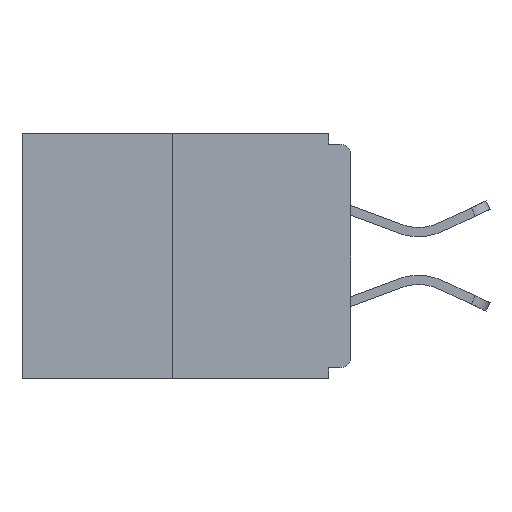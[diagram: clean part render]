
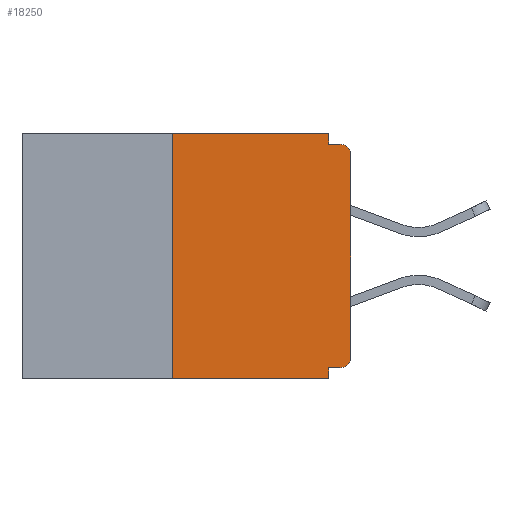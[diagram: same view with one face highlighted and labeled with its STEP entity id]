
A CAD part, left-side view. The second image highlights one B-rep face of the part: STEP entity #18250.
In plain terms, the highlighted planar face has unit normal (-1, 0, 0).
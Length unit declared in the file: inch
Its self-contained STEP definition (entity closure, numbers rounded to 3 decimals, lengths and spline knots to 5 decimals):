
#470 = CARTESIAN_POINT ( 'NONE',  ( 0., 0.46, 0. ) ) ;
#754 = AXIS2_PLACEMENT_3D ( 'NONE', #14094, #1315, #24975 ) ;
#1192 = VECTOR ( 'NONE', #9846, 39.37008 ) ;
#1315 = DIRECTION ( 'NONE',  ( -1., 0., 0. ) ) ;
#2148 = ORIENTED_EDGE ( 'NONE', *, *, #24529, .T. ) ;
#2165 = ORIENTED_EDGE ( 'NONE', *, *, #6232, .F. ) ;
#2909 = DIRECTION ( 'NONE',  ( 1., 0., 0. ) ) ;
#2956 = DIRECTION ( 'NONE',  ( 0., 1., 0. ) ) ;
#3475 = VERTEX_POINT ( 'NONE', #12424 ) ;
#3499 = CARTESIAN_POINT ( 'NONE',  ( 0., 0., 0. ) ) ;
#3639 = ORIENTED_EDGE ( 'NONE', *, *, #13414, .F. ) ;
#4383 = VERTEX_POINT ( 'NONE', #13412 ) ;
#4869 = ORIENTED_EDGE ( 'NONE', *, *, #10185, .T. ) ;
#4940 = CARTESIAN_POINT ( 'NONE',  ( 0., 0., -0.328 ) ) ;
#5083 = DIRECTION ( 'NONE',  ( 0., 0., -1. ) ) ;
#5455 = VERTEX_POINT ( 'NONE', #12194 ) ;
#5829 = CARTESIAN_POINT ( 'NONE',  ( 0., 0.015, -0.015 ) ) ;
#5889 = CARTESIAN_POINT ( 'NONE',  ( 0., 0.25, 0. ) ) ;
#6232 = EDGE_CURVE ( 'NONE', #18840, #5455, #13335, .T. ) ;
#6295 = DIRECTION ( 'NONE',  ( 0., 0., -1. ) ) ;
#6582 = CIRCLE ( 'NONE', #754, 0.015 ) ;
#6596 = EDGE_CURVE ( 'NONE', #10879, #4383, #12348, .T. ) ;
#6618 = LINE ( 'NONE', #21497, #10267 ) ;
#6805 = EDGE_CURVE ( 'NONE', #18840, #24282, #24358, .T. ) ;
#6908 = LINE ( 'NONE', #22828, #1192 ) ;
#7593 = DIRECTION ( 'NONE',  ( 0., -1., 0. ) ) ;
#7781 = LINE ( 'NONE', #3499, #22490 ) ;
#8457 = CARTESIAN_POINT ( 'NONE',  ( 0., 0.031, 0. ) ) ;
#8642 = VERTEX_POINT ( 'NONE', #5829 ) ;
#8933 = VECTOR ( 'NONE', #20960, 39.37008 ) ;
#9652 = CARTESIAN_POINT ( 'NONE',  ( 0., 0.46, 0. ) ) ;
#9846 = DIRECTION ( 'NONE',  ( 0., 0., 1. ) ) ;
#9898 = ORIENTED_EDGE ( 'NONE', *, *, #6596, .F. ) ;
#10185 = EDGE_CURVE ( 'NONE', #3475, #8642, #6582, .T. ) ;
#10267 = VECTOR ( 'NONE', #21404, 39.37008 ) ;
#10447 = VECTOR ( 'NONE', #22062, 39.37008 ) ;
#10879 = VERTEX_POINT ( 'NONE', #5889 ) ;
#11658 = VECTOR ( 'NONE', #7593, 39.37008 ) ;
#12194 = CARTESIAN_POINT ( 'NONE',  ( 0., 0.031, -0.328 ) ) ;
#12329 = CARTESIAN_POINT ( 'NONE',  ( 0., 0.031, -0.343 ) ) ;
#12348 = LINE ( 'NONE', #9652, #11658 ) ;
#12424 = CARTESIAN_POINT ( 'NONE',  ( 0., 0., -0.03 ) ) ;
#12651 = CARTESIAN_POINT ( 'NONE',  ( 0., 0.031, -0.343 ) ) ;
#12762 = FACE_OUTER_BOUND ( 'NONE', #21394, .T. ) ;
#12835 = CARTESIAN_POINT ( 'NONE',  ( 0., 0., -0.313 ) ) ;
#13335 = LINE ( 'NONE', #4940, #19704 ) ;
#13412 = CARTESIAN_POINT ( 'NONE',  ( 0., 0.031, 0. ) ) ;
#13414 = EDGE_CURVE ( 'NONE', #17838, #8642, #6618, .T. ) ;
#13547 = LINE ( 'NONE', #8457, #8933 ) ;
#14094 = CARTESIAN_POINT ( 'NONE',  ( 0., 0.015, -0.03 ) ) ;
#14880 = VERTEX_POINT ( 'NONE', #17834 ) ;
#15167 = ORIENTED_EDGE ( 'NONE', *, *, #21345, .F. ) ;
#15459 = ORIENTED_EDGE ( 'NONE', *, *, #24786, .F. ) ;
#15489 = PLANE ( 'NONE',  #16462 ) ;
#15581 = EDGE_CURVE ( 'NONE', #24282, #3475, #7781, .T. ) ;
#15740 = VECTOR ( 'NONE', #6295, 39.37008 ) ;
#15872 = DIRECTION ( 'NONE',  ( 0., 0., 1. ) ) ;
#16086 = LINE ( 'NONE', #24591, #10447 ) ;
#16462 = AXIS2_PLACEMENT_3D ( 'NONE', #470, #2909, #5083 ) ;
#16620 = CARTESIAN_POINT ( 'NONE',  ( 0., 0.015, -0.313 ) ) ;
#16723 = LINE ( 'NONE', #12329, #15740 ) ;
#17069 = ORIENTED_EDGE ( 'NONE', *, *, #15581, .T. ) ;
#17834 = CARTESIAN_POINT ( 'NONE',  ( 0., 0.25, -0.343 ) ) ;
#17838 = VERTEX_POINT ( 'NONE', #24976 ) ;
#18250 = ADVANCED_FACE ( 'NONE', ( #12762 ), #15489, .F. ) ;
#18385 = DIRECTION ( 'NONE',  ( -1., 0., 0. ) ) ;
#18568 = AXIS2_PLACEMENT_3D ( 'NONE', #16620, #18385, #18764 ) ;
#18764 = DIRECTION ( 'NONE',  ( 0., 0., -1. ) ) ;
#18840 = VERTEX_POINT ( 'NONE', #25962 ) ;
#19704 = VECTOR ( 'NONE', #2956, 39.37008 ) ;
#20960 = DIRECTION ( 'NONE',  ( 0., 0., -1. ) ) ;
#20976 = EDGE_CURVE ( 'NONE', #4383, #17838, #13547, .T. ) ;
#21345 = EDGE_CURVE ( 'NONE', #14880, #10879, #6908, .T. ) ;
#21394 = EDGE_LOOP ( 'NONE', ( #9898, #15167, #2148, #15459, #2165, #27379, #17069, #4869, #3639, #22903 ) ) ;
#21404 = DIRECTION ( 'NONE',  ( 0., -1., 0. ) ) ;
#21497 = CARTESIAN_POINT ( 'NONE',  ( 0., 0., -0.015 ) ) ;
#22062 = DIRECTION ( 'NONE',  ( 0., -1., 0. ) ) ;
#22490 = VECTOR ( 'NONE', #15872, 39.37008 ) ;
#22828 = CARTESIAN_POINT ( 'NONE',  ( 0., 0.25, 0. ) ) ;
#22903 = ORIENTED_EDGE ( 'NONE', *, *, #20976, .F. ) ;
#24282 = VERTEX_POINT ( 'NONE', #12835 ) ;
#24358 = CIRCLE ( 'NONE', #18568, 0.015 ) ;
#24529 = EDGE_CURVE ( 'NONE', #14880, #26127, #16086, .T. ) ;
#24591 = CARTESIAN_POINT ( 'NONE',  ( 0., 0.46, -0.343 ) ) ;
#24786 = EDGE_CURVE ( 'NONE', #5455, #26127, #16723, .T. ) ;
#24975 = DIRECTION ( 'NONE',  ( 0., 0., -1. ) ) ;
#24976 = CARTESIAN_POINT ( 'NONE',  ( 0., 0.031, -0.015 ) ) ;
#25962 = CARTESIAN_POINT ( 'NONE',  ( 0., 0.015, -0.328 ) ) ;
#26127 = VERTEX_POINT ( 'NONE', #12651 ) ;
#27379 = ORIENTED_EDGE ( 'NONE', *, *, #6805, .T. ) ;
